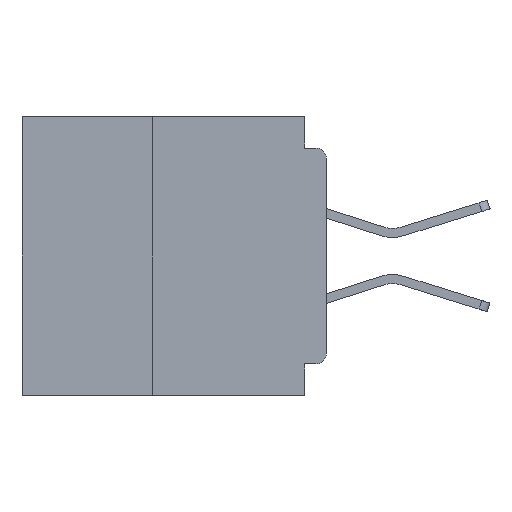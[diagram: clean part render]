
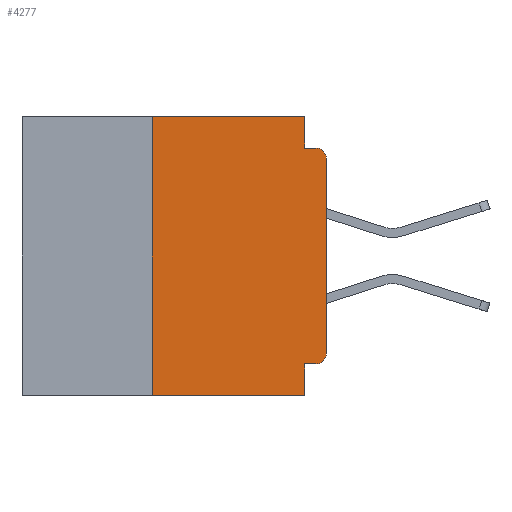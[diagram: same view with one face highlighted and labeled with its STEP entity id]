
A CAD part, left-side view. The second image highlights one B-rep face of the part: STEP entity #4277.
In plain terms, the highlighted planar face has unit normal (-1, 0, 0).
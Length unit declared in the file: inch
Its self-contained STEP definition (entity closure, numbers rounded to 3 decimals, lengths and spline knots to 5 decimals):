
#947 = EDGE_CURVE ( 'NONE', #8199, #17883, #17793, .T. ) ;
#1782 = ORIENTED_EDGE ( 'NONE', *, *, #35426, .F. ) ;
#2471 = CARTESIAN_POINT ( 'NONE',  ( 0., 0.031, -0.4 ) ) ;
#3649 = DIRECTION ( 'NONE',  ( -1., 0., 0. ) ) ;
#3945 = CARTESIAN_POINT ( 'NONE',  ( 0., 0., -0.34 ) ) ;
#3947 = CARTESIAN_POINT ( 'NONE',  ( 0., 0.25, -0.4 ) ) ;
#4250 = LINE ( 'NONE', #27848, #21113 ) ;
#4277 = ADVANCED_FACE ( 'NONE', ( #12216 ), #30850, .F. ) ;
#4353 = CARTESIAN_POINT ( 'NONE',  ( 0., 0.031, 0. ) ) ;
#4812 = CARTESIAN_POINT ( 'NONE',  ( 0., 0.015, -0.045 ) ) ;
#4947 = ORIENTED_EDGE ( 'NONE', *, *, #10590, .T. ) ;
#5649 = VECTOR ( 'NONE', #13478, 39.37008 ) ;
#6030 = DIRECTION ( 'NONE',  ( 0., 0., 1. ) ) ;
#8199 = VERTEX_POINT ( 'NONE', #40792 ) ;
#8443 = EDGE_CURVE ( 'NONE', #40597, #41664, #8641, .T. ) ;
#8641 = LINE ( 'NONE', #38740, #25487 ) ;
#8652 = LINE ( 'NONE', #13122, #43193 ) ;
#9863 = VECTOR ( 'NONE', #13188, 39.37008 ) ;
#10185 = ORIENTED_EDGE ( 'NONE', *, *, #33892, .T. ) ;
#10590 = EDGE_CURVE ( 'NONE', #32113, #14543, #13266, .T. ) ;
#11321 = CARTESIAN_POINT ( 'NONE',  ( 0., 0.015, -0.06 ) ) ;
#12216 = FACE_OUTER_BOUND ( 'NONE', #38079, .T. ) ;
#12328 = ORIENTED_EDGE ( 'NONE', *, *, #42924, .F. ) ;
#12367 = AXIS2_PLACEMENT_3D ( 'NONE', #23836, #3649, #27178 ) ;
#12826 = LINE ( 'NONE', #39600, #20715 ) ;
#13122 = CARTESIAN_POINT ( 'NONE',  ( 0., 0., -0.355 ) ) ;
#13188 = DIRECTION ( 'NONE',  ( 0., -1., 0. ) ) ;
#13260 = DIRECTION ( 'NONE',  ( 0., 1., 0. ) ) ;
#13266 = CIRCLE ( 'NONE', #12367, 0.015 ) ;
#13267 = CARTESIAN_POINT ( 'NONE',  ( 0., 0., -0.045 ) ) ;
#13478 = DIRECTION ( 'NONE',  ( 0., 0., -1. ) ) ;
#14543 = VERTEX_POINT ( 'NONE', #3945 ) ;
#14722 = DIRECTION ( 'NONE',  ( 0., 0., -1. ) ) ;
#16321 = VERTEX_POINT ( 'NONE', #27002 ) ;
#17793 = LINE ( 'NONE', #13267, #9863 ) ;
#17883 = VERTEX_POINT ( 'NONE', #4812 ) ;
#18121 = ORIENTED_EDGE ( 'NONE', *, *, #30500, .T. ) ;
#18279 = VECTOR ( 'NONE', #40003, 39.37008 ) ;
#18822 = CARTESIAN_POINT ( 'NONE',  ( 0., 0., -0.06 ) ) ;
#19483 = EDGE_CURVE ( 'NONE', #41664, #27982, #27174, .T. ) ;
#19838 = VERTEX_POINT ( 'NONE', #2471 ) ;
#20128 = CIRCLE ( 'NONE', #39852, 0.015 ) ;
#20237 = CARTESIAN_POINT ( 'NONE',  ( 0., 0.031, 0. ) ) ;
#20715 = VECTOR ( 'NONE', #6030, 39.37008 ) ;
#21113 = VECTOR ( 'NONE', #31209, 39.37008 ) ;
#21234 = CARTESIAN_POINT ( 'NONE',  ( 0., 0.437, -0.4 ) ) ;
#21782 = LINE ( 'NONE', #21234, #39531 ) ;
#22069 = CARTESIAN_POINT ( 'NONE',  ( 0., 0.015, -0.355 ) ) ;
#23256 = CARTESIAN_POINT ( 'NONE',  ( 0., 0.437, 0. ) ) ;
#23579 = LINE ( 'NONE', #20237, #5649 ) ;
#23836 = CARTESIAN_POINT ( 'NONE',  ( 0., 0.015, -0.34 ) ) ;
#25471 = ORIENTED_EDGE ( 'NONE', *, *, #33174, .T. ) ;
#25487 = VECTOR ( 'NONE', #42083, 39.37008 ) ;
#27002 = CARTESIAN_POINT ( 'NONE',  ( 0., 0.031, -0.355 ) ) ;
#27174 = LINE ( 'NONE', #23256, #18279 ) ;
#27178 = DIRECTION ( 'NONE',  ( 0., 0., -1. ) ) ;
#27848 = CARTESIAN_POINT ( 'NONE',  ( 0., 0.031, -0.4 ) ) ;
#27982 = VERTEX_POINT ( 'NONE', #4353 ) ;
#28583 = ORIENTED_EDGE ( 'NONE', *, *, #39193, .F. ) ;
#29566 = DIRECTION ( 'NONE',  ( 0., 0., -1. ) ) ;
#29710 = DIRECTION ( 'NONE',  ( 1., 0., 0. ) ) ;
#29720 = CARTESIAN_POINT ( 'NONE',  ( 0., 0.437, 0. ) ) ;
#30500 = EDGE_CURVE ( 'NONE', #14543, #36705, #12826, .T. ) ;
#30850 = PLANE ( 'NONE',  #32976 ) ;
#31171 = DIRECTION ( 'NONE',  ( 0., -1., 0. ) ) ;
#31209 = DIRECTION ( 'NONE',  ( 0., 0., -1. ) ) ;
#32113 = VERTEX_POINT ( 'NONE', #22069 ) ;
#32259 = ORIENTED_EDGE ( 'NONE', *, *, #19483, .F. ) ;
#32976 = AXIS2_PLACEMENT_3D ( 'NONE', #29720, #29710, #29566 ) ;
#33174 = EDGE_CURVE ( 'NONE', #40597, #19838, #21782, .T. ) ;
#33276 = ORIENTED_EDGE ( 'NONE', *, *, #8443, .F. ) ;
#33892 = EDGE_CURVE ( 'NONE', #36705, #17883, #20128, .T. ) ;
#34754 = DIRECTION ( 'NONE',  ( -1., 0., 0. ) ) ;
#35426 = EDGE_CURVE ( 'NONE', #16321, #19838, #4250, .T. ) ;
#36705 = VERTEX_POINT ( 'NONE', #18822 ) ;
#36902 = ORIENTED_EDGE ( 'NONE', *, *, #947, .F. ) ;
#38079 = EDGE_LOOP ( 'NONE', ( #18121, #10185, #36902, #12328, #32259, #33276, #25471, #1782, #28583, #4947 ) ) ;
#38740 = CARTESIAN_POINT ( 'NONE',  ( 0., 0.25, -0.4 ) ) ;
#39193 = EDGE_CURVE ( 'NONE', #32113, #16321, #8652, .T. ) ;
#39531 = VECTOR ( 'NONE', #31171, 39.37008 ) ;
#39600 = CARTESIAN_POINT ( 'NONE',  ( 0., 0., 0. ) ) ;
#39852 = AXIS2_PLACEMENT_3D ( 'NONE', #11321, #34754, #14722 ) ;
#40003 = DIRECTION ( 'NONE',  ( 0., -1., 0. ) ) ;
#40597 = VERTEX_POINT ( 'NONE', #3947 ) ;
#40792 = CARTESIAN_POINT ( 'NONE',  ( 0., 0.031, -0.045 ) ) ;
#41664 = VERTEX_POINT ( 'NONE', #42935 ) ;
#42083 = DIRECTION ( 'NONE',  ( 0., 0., 1. ) ) ;
#42924 = EDGE_CURVE ( 'NONE', #27982, #8199, #23579, .T. ) ;
#42935 = CARTESIAN_POINT ( 'NONE',  ( 0., 0.25, 0. ) ) ;
#43193 = VECTOR ( 'NONE', #13260, 39.37008 ) ;
